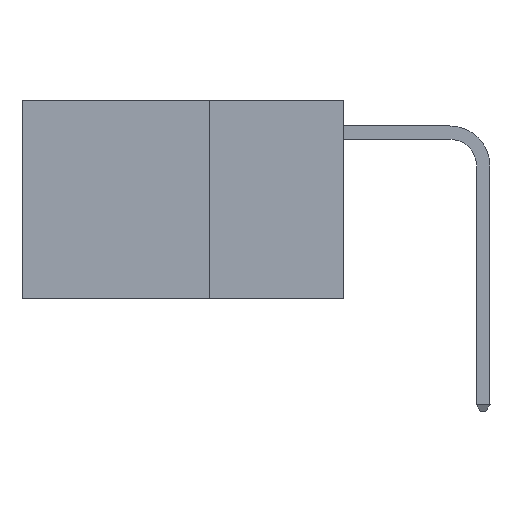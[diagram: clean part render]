
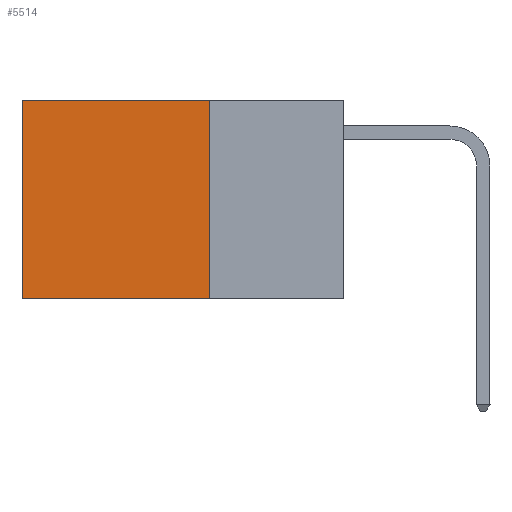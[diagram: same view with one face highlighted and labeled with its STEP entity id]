
A CAD part, left-side view. The second image highlights one B-rep face of the part: STEP entity #5514.
In plain terms, the highlighted planar face has unit normal (-1, 0, 0).
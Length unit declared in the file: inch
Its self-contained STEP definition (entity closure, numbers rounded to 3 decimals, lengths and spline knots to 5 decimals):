
#71 = VECTOR ( 'NONE', #907, 39.37008 ) ;
#791 = ORIENTED_EDGE ( 'NONE', *, *, #9483, .T. ) ;
#907 = DIRECTION ( 'NONE',  ( 0., 1., 0. ) ) ;
#1073 = DIRECTION ( 'NONE',  ( 0., 0., -1. ) ) ;
#1192 = CARTESIAN_POINT ( 'NONE',  ( 0.2625, 0.25, 0. ) ) ;
#1273 = VECTOR ( 'NONE', #1073, 39.37008 ) ;
#1599 = CARTESIAN_POINT ( 'NONE',  ( 0.2625, 0.25, 0. ) ) ;
#2024 = CARTESIAN_POINT ( 'NONE',  ( 0.2625, 0.25, 0. ) ) ;
#2548 = EDGE_CURVE ( 'NONE', #9356, #14194, #5367, .T. ) ;
#3030 = DIRECTION ( 'NONE',  ( 0., 1., 0. ) ) ;
#3061 = EDGE_CURVE ( 'NONE', #9356, #14088, #9905, .T. ) ;
#4422 = CARTESIAN_POINT ( 'NONE',  ( 0.2625, 0.25, 0. ) ) ;
#4707 = ORIENTED_EDGE ( 'NONE', *, *, #2548, .T. ) ;
#5367 = LINE ( 'NONE', #2024, #71 ) ;
#5389 = LINE ( 'NONE', #8782, #6854 ) ;
#5514 = ADVANCED_FACE ( 'NONE', ( #8223 ), #12899, .F. ) ;
#6098 = VERTEX_POINT ( 'NONE', #11739 ) ;
#6854 = VECTOR ( 'NONE', #10305, 39.37008 ) ;
#6883 = ORIENTED_EDGE ( 'NONE', *, *, #3061, .F. ) ;
#7255 = CARTESIAN_POINT ( 'NONE',  ( 0.2625, 0.25, -0.37 ) ) ;
#8223 = FACE_OUTER_BOUND ( 'NONE', #12797, .T. ) ;
#8391 = DIRECTION ( 'NONE',  ( 0., 0., -1. ) ) ;
#8616 = LINE ( 'NONE', #13210, #9262 ) ;
#8782 = CARTESIAN_POINT ( 'NONE',  ( 0.2625, 0.6, 0. ) ) ;
#9262 = VECTOR ( 'NONE', #3030, 39.37008 ) ;
#9356 = VERTEX_POINT ( 'NONE', #1192 ) ;
#9483 = EDGE_CURVE ( 'NONE', #14194, #6098, #5389, .T. ) ;
#9905 = LINE ( 'NONE', #4422, #1273 ) ;
#10202 = ORIENTED_EDGE ( 'NONE', *, *, #14321, .F. ) ;
#10305 = DIRECTION ( 'NONE',  ( 0., 0., -1. ) ) ;
#11739 = CARTESIAN_POINT ( 'NONE',  ( 0.2625, 0.6, -0.37 ) ) ;
#11772 = DIRECTION ( 'NONE',  ( 1., 0., 0. ) ) ;
#11792 = CARTESIAN_POINT ( 'NONE',  ( 0.2625, 0.6, 0. ) ) ;
#12797 = EDGE_LOOP ( 'NONE', ( #791, #10202, #6883, #4707 ) ) ;
#12899 = PLANE ( 'NONE',  #13489 ) ;
#13210 = CARTESIAN_POINT ( 'NONE',  ( 0.2625, 0.25, -0.37 ) ) ;
#13489 = AXIS2_PLACEMENT_3D ( 'NONE', #1599, #11772, #8391 ) ;
#14088 = VERTEX_POINT ( 'NONE', #7255 ) ;
#14194 = VERTEX_POINT ( 'NONE', #11792 ) ;
#14321 = EDGE_CURVE ( 'NONE', #14088, #6098, #8616, .T. ) ;
